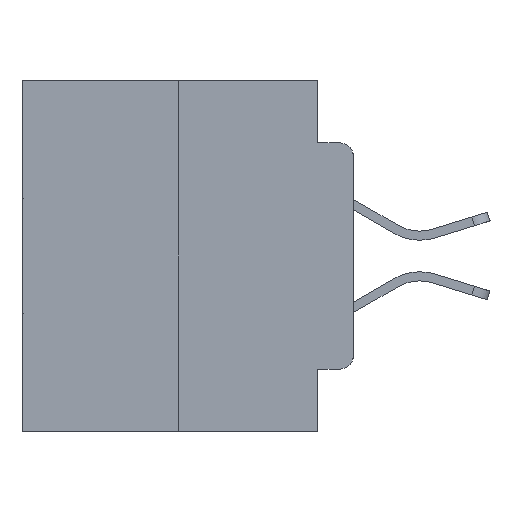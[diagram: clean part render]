
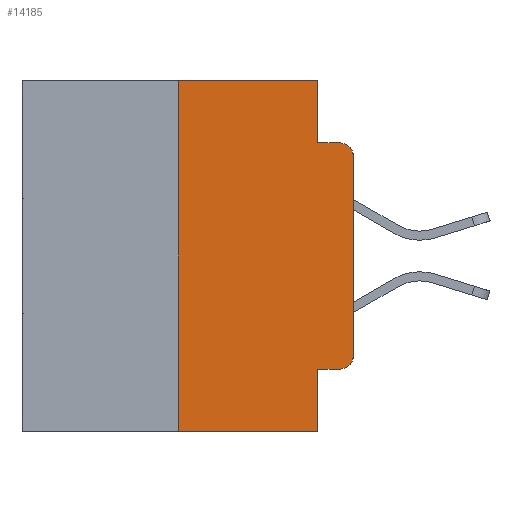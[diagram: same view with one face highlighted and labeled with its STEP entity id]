
A CAD part, left-side view. The second image highlights one B-rep face of the part: STEP entity #14185.
In plain terms, the highlighted planar face has unit normal (-1, 0, 0).
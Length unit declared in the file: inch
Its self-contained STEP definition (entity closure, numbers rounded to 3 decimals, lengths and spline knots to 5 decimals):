
#478 = CARTESIAN_POINT ( 'NONE',  ( 0., 0.02, -0.3915 ) ) ;
#977 = CARTESIAN_POINT ( 'NONE',  ( 0., 0.051, -0.0885 ) ) ;
#1604 = VERTEX_POINT ( 'NONE', #4232 ) ;
#1627 = ORIENTED_EDGE ( 'NONE', *, *, #15879, .F. ) ;
#1824 = VERTEX_POINT ( 'NONE', #9717 ) ;
#2574 = DIRECTION ( 'NONE',  ( -1., 0., 0. ) ) ;
#2575 = ORIENTED_EDGE ( 'NONE', *, *, #11932, .T. ) ;
#3163 = LINE ( 'NONE', #14361, #26129 ) ;
#3304 = EDGE_CURVE ( 'NONE', #23406, #21867, #15367, .T. ) ;
#3365 = EDGE_LOOP ( 'NONE', ( #9801, #6686, #12037, #5713, #1627, #13144, #2575, #14064, #5773, #25352 ) ) ;
#3934 = AXIS2_PLACEMENT_3D ( 'NONE', #29176, #10855, #19974 ) ;
#3989 = EDGE_CURVE ( 'NONE', #6493, #27690, #20056, .T. ) ;
#3996 = VERTEX_POINT ( 'NONE', #20792 ) ;
#4232 = CARTESIAN_POINT ( 'NONE',  ( 0., 0.051, -0.5 ) ) ;
#5126 = EDGE_CURVE ( 'NONE', #27690, #23406, #26891, .T. ) ;
#5503 = EDGE_CURVE ( 'NONE', #3996, #1604, #19292, .T. ) ;
#5713 = ORIENTED_EDGE ( 'NONE', *, *, #15190, .F. ) ;
#5773 = ORIENTED_EDGE ( 'NONE', *, *, #21262, .T. ) ;
#5848 = DIRECTION ( 'NONE',  ( 0., -1., 0. ) ) ;
#6254 = AXIS2_PLACEMENT_3D ( 'NONE', #478, #2574, #9158 ) ;
#6493 = VERTEX_POINT ( 'NONE', #24762 ) ;
#6576 = VERTEX_POINT ( 'NONE', #14494 ) ;
#6686 = ORIENTED_EDGE ( 'NONE', *, *, #3304, .T. ) ;
#7943 = DIRECTION ( 'NONE',  ( 1., 0., 0. ) ) ;
#8389 = CARTESIAN_POINT ( 'NONE',  ( 0., 0.473, 0. ) ) ;
#8496 = VECTOR ( 'NONE', #14398, 39.37008 ) ;
#9158 = DIRECTION ( 'NONE',  ( 0., 0., -1. ) ) ;
#9717 = CARTESIAN_POINT ( 'NONE',  ( 0., 0.051, 0. ) ) ;
#9801 = ORIENTED_EDGE ( 'NONE', *, *, #5126, .T. ) ;
#10091 = LINE ( 'NONE', #12620, #14126 ) ;
#10855 = DIRECTION ( 'NONE',  ( -1., 0., 0. ) ) ;
#11561 = LINE ( 'NONE', #20668, #8496 ) ;
#11779 = DIRECTION ( 'NONE',  ( 0., 0., 1. ) ) ;
#11932 = EDGE_CURVE ( 'NONE', #25647, #1604, #10091, .T. ) ;
#12037 = ORIENTED_EDGE ( 'NONE', *, *, #28451, .F. ) ;
#12260 = CARTESIAN_POINT ( 'NONE',  ( 0., 0.051, 0. ) ) ;
#12460 = VECTOR ( 'NONE', #28355, 39.37008 ) ;
#12620 = CARTESIAN_POINT ( 'NONE',  ( 0., 0.473, -0.5 ) ) ;
#13109 = EDGE_CURVE ( 'NONE', #25647, #6576, #27850, .T. ) ;
#13144 = ORIENTED_EDGE ( 'NONE', *, *, #13109, .F. ) ;
#13250 = VECTOR ( 'NONE', #11779, 39.37008 ) ;
#14064 = ORIENTED_EDGE ( 'NONE', *, *, #5503, .F. ) ;
#14126 = VECTOR ( 'NONE', #28418, 39.37008 ) ;
#14185 = ADVANCED_FACE ( 'NONE', ( #28799 ), #17364, .F. ) ;
#14361 = CARTESIAN_POINT ( 'NONE',  ( 0., 0.473, 0. ) ) ;
#14398 = DIRECTION ( 'NONE',  ( 0., 0., -1. ) ) ;
#14432 = DIRECTION ( 'NONE',  ( 0., -1., 0. ) ) ;
#14494 = CARTESIAN_POINT ( 'NONE',  ( 0., 0.25, 0. ) ) ;
#15190 = EDGE_CURVE ( 'NONE', #1824, #21380, #11561, .T. ) ;
#15367 = CIRCLE ( 'NONE', #3934, 0.02 ) ;
#15621 = VECTOR ( 'NONE', #26661, 39.37008 ) ;
#15879 = EDGE_CURVE ( 'NONE', #6576, #1824, #3163, .T. ) ;
#16262 = CARTESIAN_POINT ( 'NONE',  ( 0., 0.25, 0. ) ) ;
#17364 = PLANE ( 'NONE',  #26588 ) ;
#18305 = VECTOR ( 'NONE', #14432, 39.37008 ) ;
#18659 = VECTOR ( 'NONE', #20373, 39.37008 ) ;
#18719 = CARTESIAN_POINT ( 'NONE',  ( 0., 0., -0.1085 ) ) ;
#19292 = LINE ( 'NONE', #12260, #12460 ) ;
#19735 = DIRECTION ( 'NONE',  ( 0., 0., -1. ) ) ;
#19974 = DIRECTION ( 'NONE',  ( 0., 0., -1. ) ) ;
#20056 = CIRCLE ( 'NONE', #6254, 0.02 ) ;
#20373 = DIRECTION ( 'NONE',  ( 0., 0., 1. ) ) ;
#20668 = CARTESIAN_POINT ( 'NONE',  ( 0., 0.051, 0. ) ) ;
#20792 = CARTESIAN_POINT ( 'NONE',  ( 0., 0.051, -0.4115 ) ) ;
#21262 = EDGE_CURVE ( 'NONE', #3996, #6493, #22631, .T. ) ;
#21380 = VERTEX_POINT ( 'NONE', #29206 ) ;
#21867 = VERTEX_POINT ( 'NONE', #24806 ) ;
#22631 = LINE ( 'NONE', #26946, #15621 ) ;
#23406 = VERTEX_POINT ( 'NONE', #18719 ) ;
#24324 = CARTESIAN_POINT ( 'NONE',  ( 0., 0., -0.3915 ) ) ;
#24762 = CARTESIAN_POINT ( 'NONE',  ( 0., 0.02, -0.4115 ) ) ;
#24806 = CARTESIAN_POINT ( 'NONE',  ( 0., 0.02, -0.0885 ) ) ;
#24924 = CARTESIAN_POINT ( 'NONE',  ( 0., 0., 0. ) ) ;
#25352 = ORIENTED_EDGE ( 'NONE', *, *, #3989, .T. ) ;
#25647 = VERTEX_POINT ( 'NONE', #27399 ) ;
#26129 = VECTOR ( 'NONE', #5848, 39.37008 ) ;
#26588 = AXIS2_PLACEMENT_3D ( 'NONE', #8389, #7943, #19735 ) ;
#26661 = DIRECTION ( 'NONE',  ( 0., -1., 0. ) ) ;
#26891 = LINE ( 'NONE', #24924, #18659 ) ;
#26946 = CARTESIAN_POINT ( 'NONE',  ( 0., 0.051, -0.4115 ) ) ;
#27399 = CARTESIAN_POINT ( 'NONE',  ( 0., 0.25, -0.5 ) ) ;
#27690 = VERTEX_POINT ( 'NONE', #24324 ) ;
#27814 = LINE ( 'NONE', #977, #18305 ) ;
#27850 = LINE ( 'NONE', #16262, #13250 ) ;
#28355 = DIRECTION ( 'NONE',  ( 0., 0., -1. ) ) ;
#28418 = DIRECTION ( 'NONE',  ( 0., -1., 0. ) ) ;
#28451 = EDGE_CURVE ( 'NONE', #21380, #21867, #27814, .T. ) ;
#28799 = FACE_OUTER_BOUND ( 'NONE', #3365, .T. ) ;
#29176 = CARTESIAN_POINT ( 'NONE',  ( 0., 0.02, -0.1085 ) ) ;
#29206 = CARTESIAN_POINT ( 'NONE',  ( 0., 0.051, -0.0885 ) ) ;
